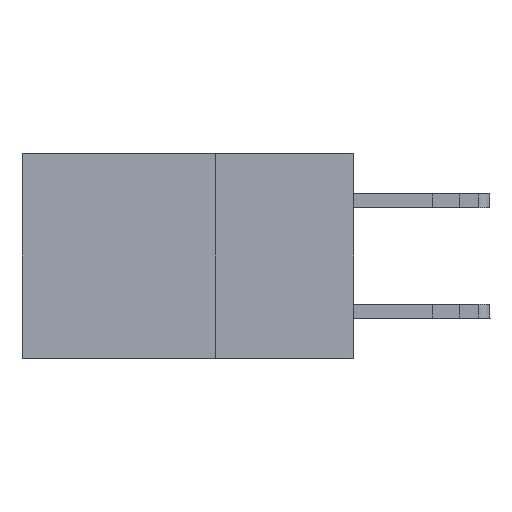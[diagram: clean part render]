
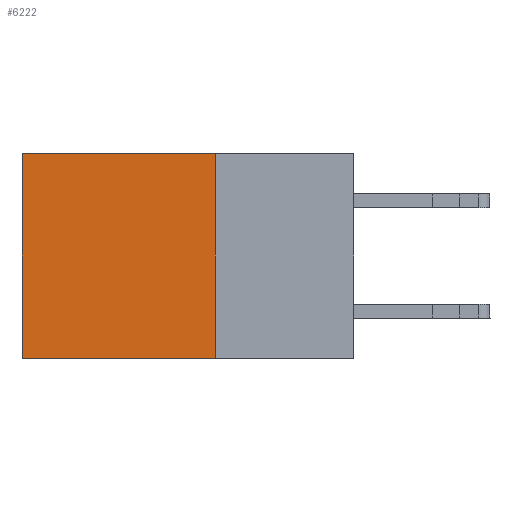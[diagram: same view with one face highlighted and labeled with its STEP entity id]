
A CAD part, left-side view. The second image highlights one B-rep face of the part: STEP entity #6222.
In plain terms, the highlighted planar face has unit normal (-1, 0, 0).
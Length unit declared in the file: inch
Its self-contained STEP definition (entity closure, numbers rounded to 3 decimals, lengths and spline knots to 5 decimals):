
#69 = VERTEX_POINT ( 'NONE', #14560 ) ;
#81 = FACE_OUTER_BOUND ( 'NONE', #5254, .T. ) ;
#327 = CARTESIAN_POINT ( 'NONE',  ( 0.2875, 0.25, 0. ) ) ;
#551 = CARTESIAN_POINT ( 'NONE',  ( 0.2875, 0.25, -0.37 ) ) ;
#983 = EDGE_CURVE ( 'NONE', #1792, #69, #1780, .T. ) ;
#1568 = ORIENTED_EDGE ( 'NONE', *, *, #7562, .F. ) ;
#1780 = LINE ( 'NONE', #14507, #6900 ) ;
#1792 = VERTEX_POINT ( 'NONE', #551 ) ;
#2035 = ORIENTED_EDGE ( 'NONE', *, *, #983, .F. ) ;
#2849 = ORIENTED_EDGE ( 'NONE', *, *, #6499, .T. ) ;
#3261 = LINE ( 'NONE', #12441, #11218 ) ;
#4694 = DIRECTION ( 'NONE',  ( 0., 1., 0. ) ) ;
#4922 = CARTESIAN_POINT ( 'NONE',  ( 0.2875, 0.25, 0. ) ) ;
#5254 = EDGE_LOOP ( 'NONE', ( #5593, #2035, #1568, #2849 ) ) ;
#5340 = CARTESIAN_POINT ( 'NONE',  ( 0.2875, 0.6, 0. ) ) ;
#5593 = ORIENTED_EDGE ( 'NONE', *, *, #11044, .T. ) ;
#5827 = VECTOR ( 'NONE', #11841, 39.37008 ) ;
#6222 = ADVANCED_FACE ( 'NONE', ( #81 ), #15509, .F. ) ;
#6499 = EDGE_CURVE ( 'NONE', #9986, #7522, #8593, .T. ) ;
#6519 = CARTESIAN_POINT ( 'NONE',  ( 0.2875, 0.25, 0. ) ) ;
#6900 = VECTOR ( 'NONE', #6934, 39.37008 ) ;
#6934 = DIRECTION ( 'NONE',  ( 0., 1., 0. ) ) ;
#7522 = VERTEX_POINT ( 'NONE', #5340 ) ;
#7562 = EDGE_CURVE ( 'NONE', #9986, #1792, #10385, .T. ) ;
#8092 = DIRECTION ( 'NONE',  ( 1., 0., 0. ) ) ;
#8593 = LINE ( 'NONE', #12463, #15484 ) ;
#8652 = DIRECTION ( 'NONE',  ( 0., 0., -1. ) ) ;
#9986 = VERTEX_POINT ( 'NONE', #4922 ) ;
#10385 = LINE ( 'NONE', #6519, #5827 ) ;
#10951 = DIRECTION ( 'NONE',  ( 0., 0., -1. ) ) ;
#11044 = EDGE_CURVE ( 'NONE', #7522, #69, #3261, .T. ) ;
#11218 = VECTOR ( 'NONE', #8652, 39.37008 ) ;
#11841 = DIRECTION ( 'NONE',  ( 0., 0., -1. ) ) ;
#12441 = CARTESIAN_POINT ( 'NONE',  ( 0.2875, 0.6, 0. ) ) ;
#12463 = CARTESIAN_POINT ( 'NONE',  ( 0.2875, 0.25, 0. ) ) ;
#14145 = AXIS2_PLACEMENT_3D ( 'NONE', #327, #8092, #10951 ) ;
#14507 = CARTESIAN_POINT ( 'NONE',  ( 0.2875, 0.25, -0.37 ) ) ;
#14560 = CARTESIAN_POINT ( 'NONE',  ( 0.2875, 0.6, -0.37 ) ) ;
#15484 = VECTOR ( 'NONE', #4694, 39.37008 ) ;
#15509 = PLANE ( 'NONE',  #14145 ) ;
